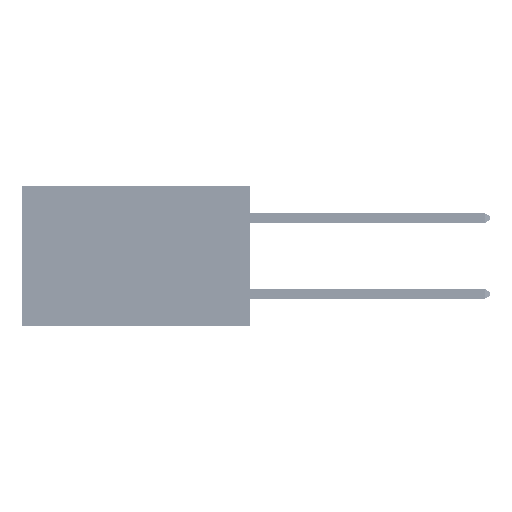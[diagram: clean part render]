
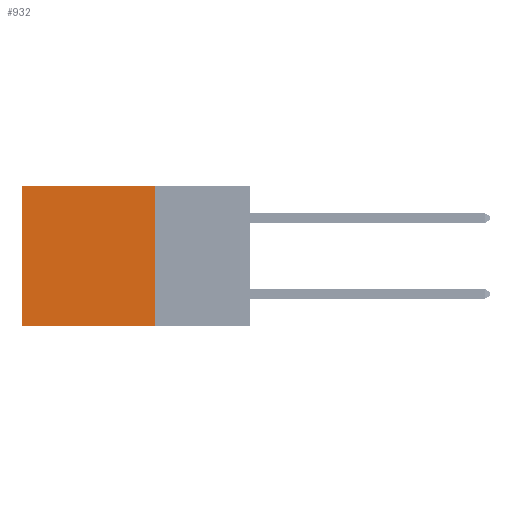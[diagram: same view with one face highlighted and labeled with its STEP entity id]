
A CAD part, left-side view. The second image highlights one B-rep face of the part: STEP entity #932.
In plain terms, the highlighted planar face has unit normal (-1, 0, 0).
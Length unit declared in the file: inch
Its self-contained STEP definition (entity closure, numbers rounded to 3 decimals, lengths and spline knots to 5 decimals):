
#647 = DIRECTION ( 'NONE',  ( 0., 0., -1. ) ) ;
#932 = ADVANCED_FACE ( 'NONE', ( #13116 ), #16520, .F. ) ;
#3020 = CARTESIAN_POINT ( 'NONE',  ( 0.2875, 0.25, -0.37 ) ) ;
#4227 = VECTOR ( 'NONE', #34266, 39.37008 ) ;
#5857 = EDGE_CURVE ( 'NONE', #25584, #46734, #19898, .T. ) ;
#9973 = VERTEX_POINT ( 'NONE', #48338 ) ;
#10164 = CARTESIAN_POINT ( 'NONE',  ( 0.2875, 0.6, 0. ) ) ;
#11772 = AXIS2_PLACEMENT_3D ( 'NONE', #48612, #44569, #647 ) ;
#12406 = EDGE_CURVE ( 'NONE', #35062, #9973, #41843, .T. ) ;
#13116 = FACE_OUTER_BOUND ( 'NONE', #15577, .T. ) ;
#13988 = CARTESIAN_POINT ( 'NONE',  ( 0.2875, 0.25, 0. ) ) ;
#15577 = EDGE_LOOP ( 'NONE', ( #36468, #46149, #41573, #43362 ) ) ;
#16520 = PLANE ( 'NONE',  #11772 ) ;
#19898 = LINE ( 'NONE', #30196, #4227 ) ;
#23140 = DIRECTION ( 'NONE',  ( 0., 1., 0. ) ) ;
#23386 = DIRECTION ( 'NONE',  ( 0., 0., -1. ) ) ;
#25172 = EDGE_CURVE ( 'NONE', #9973, #46734, #47771, .T. ) ;
#25584 = VERTEX_POINT ( 'NONE', #10164 ) ;
#26234 = DIRECTION ( 'NONE',  ( 0., 1., 0. ) ) ;
#26756 = VECTOR ( 'NONE', #23386, 39.37008 ) ;
#29137 = CARTESIAN_POINT ( 'NONE',  ( 0.2875, 0.25, 0. ) ) ;
#30196 = CARTESIAN_POINT ( 'NONE',  ( 0.2875, 0.6, 0. ) ) ;
#32093 = VECTOR ( 'NONE', #23140, 39.37008 ) ;
#33307 = EDGE_CURVE ( 'NONE', #35062, #25584, #43693, .T. ) ;
#34266 = DIRECTION ( 'NONE',  ( 0., 0., -1. ) ) ;
#35062 = VERTEX_POINT ( 'NONE', #29137 ) ;
#36468 = ORIENTED_EDGE ( 'NONE', *, *, #5857, .T. ) ;
#38890 = CARTESIAN_POINT ( 'NONE',  ( 0.2875, 0.25, 0. ) ) ;
#40624 = VECTOR ( 'NONE', #26234, 39.37008 ) ;
#41573 = ORIENTED_EDGE ( 'NONE', *, *, #12406, .F. ) ;
#41843 = LINE ( 'NONE', #38890, #26756 ) ;
#43362 = ORIENTED_EDGE ( 'NONE', *, *, #33307, .T. ) ;
#43693 = LINE ( 'NONE', #13988, #40624 ) ;
#44569 = DIRECTION ( 'NONE',  ( 1., 0., 0. ) ) ;
#46149 = ORIENTED_EDGE ( 'NONE', *, *, #25172, .F. ) ;
#46734 = VERTEX_POINT ( 'NONE', #49486 ) ;
#47771 = LINE ( 'NONE', #3020, #32093 ) ;
#48338 = CARTESIAN_POINT ( 'NONE',  ( 0.2875, 0.25, -0.37 ) ) ;
#48612 = CARTESIAN_POINT ( 'NONE',  ( 0.2875, 0.25, 0. ) ) ;
#49486 = CARTESIAN_POINT ( 'NONE',  ( 0.2875, 0.6, -0.37 ) ) ;
